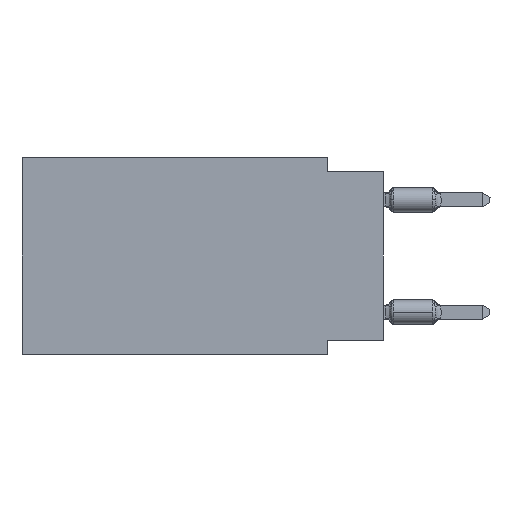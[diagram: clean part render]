
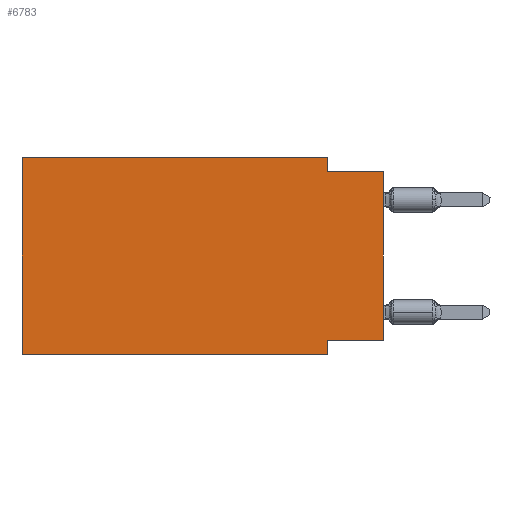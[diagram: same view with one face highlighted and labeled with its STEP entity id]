
A CAD part, left-side view. The second image highlights one B-rep face of the part: STEP entity #6783.
In plain terms, the highlighted planar face has unit normal (-1, 0, 0).
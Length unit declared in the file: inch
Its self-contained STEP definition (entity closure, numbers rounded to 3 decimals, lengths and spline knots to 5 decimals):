
#299 = ORIENTED_EDGE ( 'NONE', *, *, #5894, .F. ) ;
#530 = DIRECTION ( 'NONE',  ( 0., 1., 0. ) ) ;
#1548 = VERTEX_POINT ( 'NONE', #4417 ) ;
#1722 = CARTESIAN_POINT ( 'NONE',  ( 0., 0.645, 0. ) ) ;
#2316 = CARTESIAN_POINT ( 'NONE',  ( 0., 0.1, -0.325 ) ) ;
#2323 = CARTESIAN_POINT ( 'NONE',  ( 0., 0.1, -0.35 ) ) ;
#2655 = CARTESIAN_POINT ( 'NONE',  ( 0., 0.645, 0. ) ) ;
#3333 = EDGE_CURVE ( 'NONE', #1548, #5981, #7404, .T. ) ;
#4095 = LINE ( 'NONE', #20592, #18207 ) ;
#4178 = VECTOR ( 'NONE', #530, 39.37008 ) ;
#4417 = CARTESIAN_POINT ( 'NONE',  ( 0., 0., -0.325 ) ) ;
#4656 = VERTEX_POINT ( 'NONE', #17079 ) ;
#4823 = LINE ( 'NONE', #24895, #21661 ) ;
#5228 = LINE ( 'NONE', #23842, #20233 ) ;
#5599 = ORIENTED_EDGE ( 'NONE', *, *, #11902, .F. ) ;
#5629 = DIRECTION ( 'NONE',  ( 0., 0., 1. ) ) ;
#5807 = CARTESIAN_POINT ( 'NONE',  ( 0., 0., 0. ) ) ;
#5894 = EDGE_CURVE ( 'NONE', #1548, #16260, #10601, .T. ) ;
#5981 = VERTEX_POINT ( 'NONE', #20333 ) ;
#6322 = LINE ( 'NONE', #22550, #25051 ) ;
#6328 = VERTEX_POINT ( 'NONE', #16270 ) ;
#6463 = DIRECTION ( 'NONE',  ( 0., 0., -1. ) ) ;
#6783 = ADVANCED_FACE ( 'NONE', ( #13978 ), #26225, .F. ) ;
#7404 = LINE ( 'NONE', #5807, #18026 ) ;
#7825 = DIRECTION ( 'NONE',  ( 0., -1., 0. ) ) ;
#7995 = CARTESIAN_POINT ( 'NONE',  ( 0., 0.645, 0. ) ) ;
#8791 = DIRECTION ( 'NONE',  ( 0., 0., -1. ) ) ;
#9062 = EDGE_LOOP ( 'NONE', ( #25274, #13008, #17059, #26161, #23506, #24446, #5599, #299 ) ) ;
#10601 = LINE ( 'NONE', #18725, #4178 ) ;
#10857 = VECTOR ( 'NONE', #21844, 39.37008 ) ;
#11478 = CARTESIAN_POINT ( 'NONE',  ( 0., 0., -0.025 ) ) ;
#11623 = EDGE_CURVE ( 'NONE', #24874, #6328, #6322, .T. ) ;
#11902 = EDGE_CURVE ( 'NONE', #16260, #23293, #4823, .T. ) ;
#13008 = ORIENTED_EDGE ( 'NONE', *, *, #23538, .F. ) ;
#13978 = FACE_OUTER_BOUND ( 'NONE', #9062, .T. ) ;
#14110 = DIRECTION ( 'NONE',  ( 1., 0., 0. ) ) ;
#14207 = EDGE_CURVE ( 'NONE', #4656, #23293, #4095, .T. ) ;
#15382 = EDGE_CURVE ( 'NONE', #22336, #24874, #17941, .T. ) ;
#16260 = VERTEX_POINT ( 'NONE', #2316 ) ;
#16270 = CARTESIAN_POINT ( 'NONE',  ( 0., 0.1, -0.025 ) ) ;
#16990 = VECTOR ( 'NONE', #7825, 39.37008 ) ;
#17059 = ORIENTED_EDGE ( 'NONE', *, *, #11623, .F. ) ;
#17079 = CARTESIAN_POINT ( 'NONE',  ( 0., 0.645, -0.35 ) ) ;
#17592 = EDGE_CURVE ( 'NONE', #4656, #22336, #5228, .T. ) ;
#17941 = LINE ( 'NONE', #1722, #16990 ) ;
#18026 = VECTOR ( 'NONE', #25752, 39.37008 ) ;
#18207 = VECTOR ( 'NONE', #22581, 39.37008 ) ;
#18725 = CARTESIAN_POINT ( 'NONE',  ( 0., 0., -0.325 ) ) ;
#20233 = VECTOR ( 'NONE', #5629, 39.37008 ) ;
#20333 = CARTESIAN_POINT ( 'NONE',  ( 0., 0., -0.025 ) ) ;
#20479 = LINE ( 'NONE', #11478, #10857 ) ;
#20592 = CARTESIAN_POINT ( 'NONE',  ( 0., 0.645, -0.35 ) ) ;
#20868 = CARTESIAN_POINT ( 'NONE',  ( 0., 0.1, 0. ) ) ;
#21661 = VECTOR ( 'NONE', #8791, 39.37008 ) ;
#21844 = DIRECTION ( 'NONE',  ( 0., -1., 0. ) ) ;
#22250 = DIRECTION ( 'NONE',  ( 0., 0., -1. ) ) ;
#22336 = VERTEX_POINT ( 'NONE', #2655 ) ;
#22550 = CARTESIAN_POINT ( 'NONE',  ( 0., 0.1, 0. ) ) ;
#22581 = DIRECTION ( 'NONE',  ( 0., -1., 0. ) ) ;
#23293 = VERTEX_POINT ( 'NONE', #2323 ) ;
#23506 = ORIENTED_EDGE ( 'NONE', *, *, #17592, .F. ) ;
#23538 = EDGE_CURVE ( 'NONE', #6328, #5981, #20479, .T. ) ;
#23842 = CARTESIAN_POINT ( 'NONE',  ( 0., 0.645, 0. ) ) ;
#24446 = ORIENTED_EDGE ( 'NONE', *, *, #14207, .T. ) ;
#24595 = AXIS2_PLACEMENT_3D ( 'NONE', #7995, #14110, #22250 ) ;
#24874 = VERTEX_POINT ( 'NONE', #20868 ) ;
#24895 = CARTESIAN_POINT ( 'NONE',  ( 0., 0.1, -0.35 ) ) ;
#25051 = VECTOR ( 'NONE', #6463, 39.37008 ) ;
#25274 = ORIENTED_EDGE ( 'NONE', *, *, #3333, .T. ) ;
#25752 = DIRECTION ( 'NONE',  ( 0., 0., 1. ) ) ;
#26161 = ORIENTED_EDGE ( 'NONE', *, *, #15382, .F. ) ;
#26225 = PLANE ( 'NONE',  #24595 ) ;
